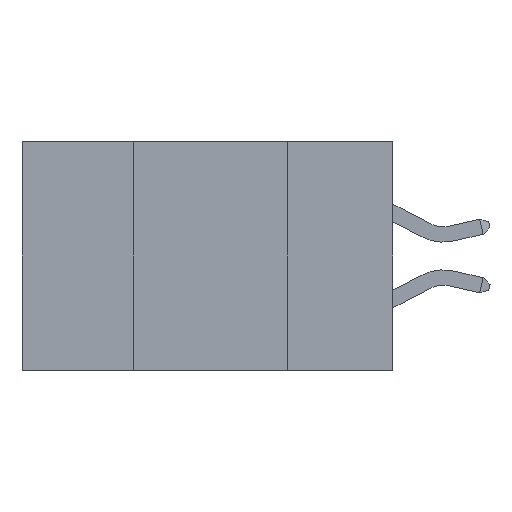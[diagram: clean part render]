
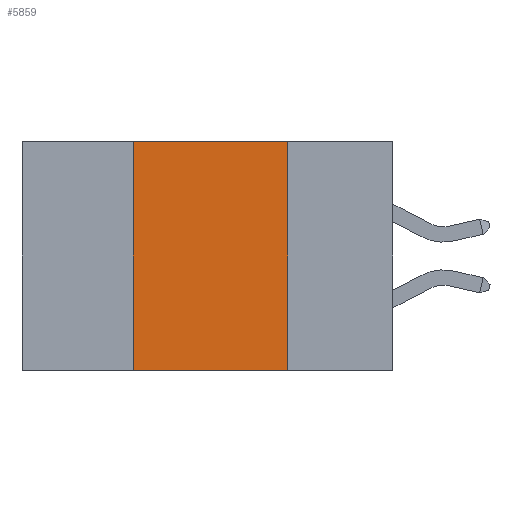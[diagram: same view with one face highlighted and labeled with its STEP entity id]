
A CAD part, left-side view. The second image highlights one B-rep face of the part: STEP entity #5859.
In plain terms, the highlighted planar face has unit normal (-1, 0, 0).
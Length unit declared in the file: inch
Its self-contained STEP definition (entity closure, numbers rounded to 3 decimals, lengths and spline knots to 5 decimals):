
#391 = CARTESIAN_POINT ( 'NONE',  ( 0., 0.17, 0. ) ) ;
#2088 = DIRECTION ( 'NONE',  ( 0., 0., -1. ) ) ;
#2262 = DIRECTION ( 'NONE',  ( 0., 0., -1. ) ) ;
#2889 = LINE ( 'NONE', #16760, #4409 ) ;
#4255 = LINE ( 'NONE', #391, #24555 ) ;
#4409 = VECTOR ( 'NONE', #19696, 39.37008 ) ;
#5104 = ORIENTED_EDGE ( 'NONE', *, *, #10759, .F. ) ;
#5435 = CARTESIAN_POINT ( 'NONE',  ( 0., 0.6, 0. ) ) ;
#5859 = ADVANCED_FACE ( 'NONE', ( #7347 ), #21515, .F. ) ;
#7347 = FACE_OUTER_BOUND ( 'NONE', #17181, .T. ) ;
#9215 = CARTESIAN_POINT ( 'NONE',  ( 0., 0.6, 0. ) ) ;
#9310 = DIRECTION ( 'NONE',  ( 0., -1., 0. ) ) ;
#10759 = EDGE_CURVE ( 'NONE', #22181, #23601, #20544, .T. ) ;
#12283 = LINE ( 'NONE', #15440, #18776 ) ;
#12459 = ORIENTED_EDGE ( 'NONE', *, *, #24904, .F. ) ;
#13436 = VECTOR ( 'NONE', #9310, 39.37008 ) ;
#14334 = EDGE_CURVE ( 'NONE', #17177, #22181, #12283, .T. ) ;
#14822 = CARTESIAN_POINT ( 'NONE',  ( 0., 0.42, -0.37 ) ) ;
#15143 = DIRECTION ( 'NONE',  ( 1., 0., 0. ) ) ;
#15440 = CARTESIAN_POINT ( 'NONE',  ( 0., 0.42, 0. ) ) ;
#16760 = CARTESIAN_POINT ( 'NONE',  ( 0., 0.6, -0.37 ) ) ;
#16858 = CARTESIAN_POINT ( 'NONE',  ( 0., 0.42, 0. ) ) ;
#16994 = AXIS2_PLACEMENT_3D ( 'NONE', #9215, #15143, #2088 ) ;
#17177 = VERTEX_POINT ( 'NONE', #14822 ) ;
#17181 = EDGE_LOOP ( 'NONE', ( #12459, #5104, #19611, #20818 ) ) ;
#18776 = VECTOR ( 'NONE', #25277, 39.37008 ) ;
#19611 = ORIENTED_EDGE ( 'NONE', *, *, #14334, .F. ) ;
#19696 = DIRECTION ( 'NONE',  ( 0., -1., 0. ) ) ;
#20544 = LINE ( 'NONE', #5435, #13436 ) ;
#20736 = CARTESIAN_POINT ( 'NONE',  ( 0., 0.17, -0.37 ) ) ;
#20818 = ORIENTED_EDGE ( 'NONE', *, *, #20849, .T. ) ;
#20849 = EDGE_CURVE ( 'NONE', #17177, #22838, #2889, .T. ) ;
#21515 = PLANE ( 'NONE',  #16994 ) ;
#22181 = VERTEX_POINT ( 'NONE', #16858 ) ;
#22346 = CARTESIAN_POINT ( 'NONE',  ( 0., 0.17, 0. ) ) ;
#22838 = VERTEX_POINT ( 'NONE', #20736 ) ;
#23601 = VERTEX_POINT ( 'NONE', #22346 ) ;
#24555 = VECTOR ( 'NONE', #2262, 39.37008 ) ;
#24904 = EDGE_CURVE ( 'NONE', #23601, #22838, #4255, .T. ) ;
#25277 = DIRECTION ( 'NONE',  ( 0., 0., 1. ) ) ;
